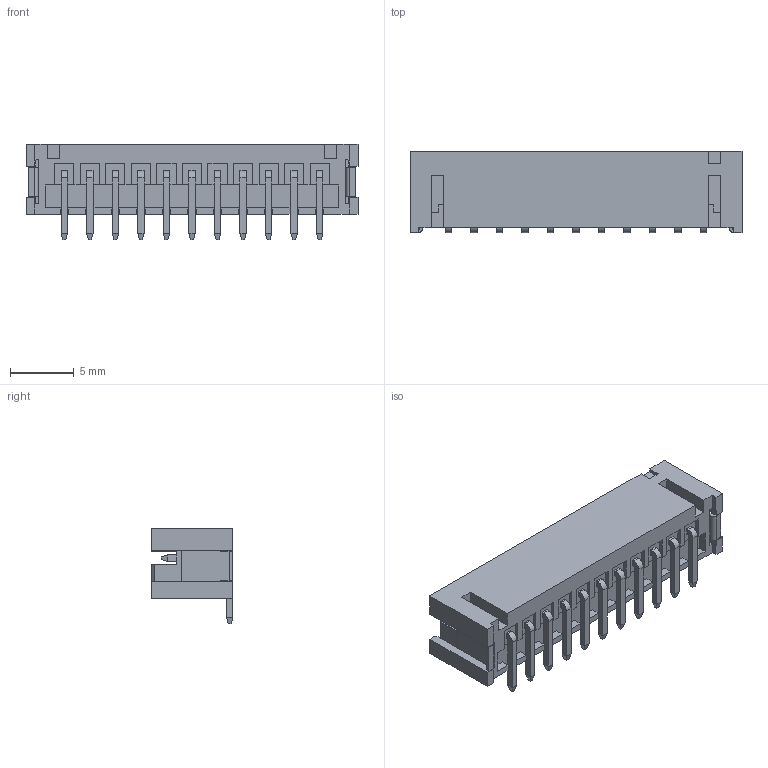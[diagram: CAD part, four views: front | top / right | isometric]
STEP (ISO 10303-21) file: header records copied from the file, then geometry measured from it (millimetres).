
FILE_DESCRIPTION (( 'STEP AP203' ), '1' );
FILE_NAME ('140-511-417-011.STEP', '2020-03-31T20:05:48', ( '' ), ( '' ), 'SwSTEP 2.0', 'SolidWorks 2016', '' );
FILE_SCHEMA (( 'CONFIG_CONTROL_DESIGN' ));
Length unit declared in the file: millimetre
Products named in the file (4): V SMT Contact; V SMT Housing_511; V SMT Pad; 140-511-417-011
Assembly tree (14 placements, depth 2):
  140-511-417-011
    V SMT Housing_511
    V SMT Contact  x11
    V SMT Pad  x2
Bounding box: 26 x 6.4 x 7.5 mm (x, y, z)
Volume: 377.2 mm3; surface area: 1364 mm2
Topology: 14 solids, 14 shells, 518 faces, 1296 edges, 802 vertices
Faces by surface type: plane 492, cylinder 26
Entity records: 9922 total; most frequent: CARTESIAN_POINT 1659, ORIENTED_EDGE 1640, DIRECTION 1430, EDGE_CURVE 820, LINE 812, VECTOR 812, VERTEX_POINT 538, AXIS2_PLACEMENT_3D 309
